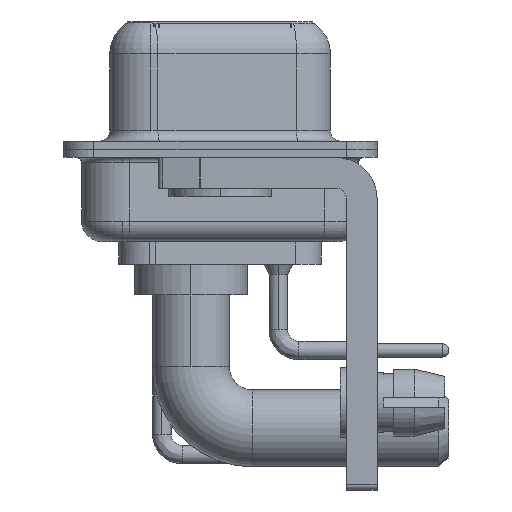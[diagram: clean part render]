
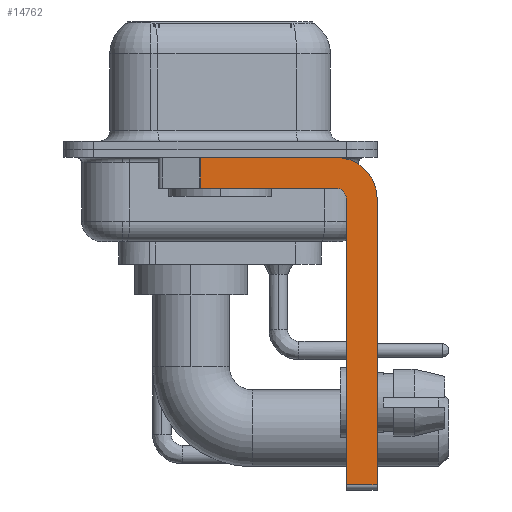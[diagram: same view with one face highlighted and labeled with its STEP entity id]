
A CAD part, left-side view. The second image highlights one B-rep face of the part: STEP entity #14762.
In plain terms, the highlighted planar face has unit normal (-1, 0, 0).
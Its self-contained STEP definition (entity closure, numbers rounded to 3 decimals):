
#224 = LINE ( 'NONE', #16806, #29640 ) ;
#698 = EDGE_CURVE ( 'NONE', #21235, #27137, #23874, .T. ) ;
#799 = ORIENTED_EDGE ( 'NONE', *, *, #13744, .F. ) ;
#1162 = EDGE_CURVE ( 'NONE', #33202, #16290, #27700, .T. ) ;
#1619 = AXIS2_PLACEMENT_3D ( 'NONE', #22233, #13235, #7358 ) ;
#1814 = ORIENTED_EDGE ( 'NONE', *, *, #33351, .T. ) ;
#1931 = CARTESIAN_POINT ( 'NONE',  ( -2.9, -5.65, -1.9 ) ) ;
#2592 = CARTESIAN_POINT ( 'NONE',  ( -2.9, -7.65, -2.4 ) ) ;
#2836 = CARTESIAN_POINT ( 'NONE',  ( -2.9, 0.978, -1.9 ) ) ;
#4672 = VECTOR ( 'NONE', #6950, 1000. ) ;
#6358 = VERTEX_POINT ( 'NONE', #12245 ) ;
#6875 = CARTESIAN_POINT ( 'NONE',  ( -2.9, -6.15, -16.35 ) ) ;
#6950 = DIRECTION ( 'NONE',  ( 0., 1., 0. ) ) ;
#7358 = DIRECTION ( 'NONE',  ( 0., 0., -1. ) ) ;
#7416 = DIRECTION ( 'NONE',  ( 0., -1., 0. ) ) ;
#8097 = VERTEX_POINT ( 'NONE', #25454 ) ;
#8476 = AXIS2_PLACEMENT_3D ( 'NONE', #9347, #26274, #34347 ) ;
#9347 = CARTESIAN_POINT ( 'NONE',  ( -2.9, -5.65, -2.4 ) ) ;
#10268 = EDGE_CURVE ( 'NONE', #16290, #21235, #20741, .T. ) ;
#10754 = VECTOR ( 'NONE', #27327, 1000. ) ;
#11011 = FACE_OUTER_BOUND ( 'NONE', #13887, .T. ) ;
#11871 = DIRECTION ( 'NONE',  ( 0., -1., 0. ) ) ;
#12245 = CARTESIAN_POINT ( 'NONE',  ( -2.9, 0.978, -0.4 ) ) ;
#12428 = EDGE_CURVE ( 'NONE', #6358, #27137, #224, .T. ) ;
#13235 = DIRECTION ( 'NONE',  ( 1., 0., 0. ) ) ;
#13590 = EDGE_CURVE ( 'NONE', #24526, #23836, #19670, .T. ) ;
#13744 = EDGE_CURVE ( 'NONE', #8097, #24526, #24337, .T. ) ;
#13887 = EDGE_LOOP ( 'NONE', ( #33103, #19713, #18801, #13941, #35571, #1814, #21103, #799 ) ) ;
#13941 = ORIENTED_EDGE ( 'NONE', *, *, #10268, .F. ) ;
#14249 = AXIS2_PLACEMENT_3D ( 'NONE', #33777, #14308, #25518 ) ;
#14308 = DIRECTION ( 'NONE',  ( -1., 0., 0. ) ) ;
#14762 = ADVANCED_FACE ( 'NONE', ( #11011 ), #27752, .F. ) ;
#16290 = VERTEX_POINT ( 'NONE', #27798 ) ;
#16806 = CARTESIAN_POINT ( 'NONE',  ( -2.9, 0.978, -1.9 ) ) ;
#17212 = LINE ( 'NONE', #22878, #17606 ) ;
#17606 = VECTOR ( 'NONE', #11871, 1000. ) ;
#18801 = ORIENTED_EDGE ( 'NONE', *, *, #698, .F. ) ;
#19670 = LINE ( 'NONE', #31049, #31983 ) ;
#19713 = ORIENTED_EDGE ( 'NONE', *, *, #12428, .T. ) ;
#20741 = CIRCLE ( 'NONE', #14249, 0.5 ) ;
#21103 = ORIENTED_EDGE ( 'NONE', *, *, #13590, .F. ) ;
#21235 = VERTEX_POINT ( 'NONE', #1931 ) ;
#21413 = LINE ( 'NONE', #32612, #25552 ) ;
#22233 = CARTESIAN_POINT ( 'NONE',  ( -2.9, -5.65, -2.4 ) ) ;
#22878 = CARTESIAN_POINT ( 'NONE',  ( -2.9, 3., -0.4 ) ) ;
#23836 = VERTEX_POINT ( 'NONE', #28754 ) ;
#23874 = LINE ( 'NONE', #29037, #4672 ) ;
#24337 = CIRCLE ( 'NONE', #8476, 2. ) ;
#24526 = VERTEX_POINT ( 'NONE', #2592 ) ;
#24767 = CARTESIAN_POINT ( 'NONE',  ( -2.9, -6.15, -16.6 ) ) ;
#25454 = CARTESIAN_POINT ( 'NONE',  ( -2.9, -5.65, -0.4 ) ) ;
#25518 = DIRECTION ( 'NONE',  ( 0., 0., 1. ) ) ;
#25552 = VECTOR ( 'NONE', #7416, 1000. ) ;
#25898 = EDGE_CURVE ( 'NONE', #6358, #8097, #17212, .T. ) ;
#26274 = DIRECTION ( 'NONE',  ( 1., 0., 0. ) ) ;
#27137 = VERTEX_POINT ( 'NONE', #2836 ) ;
#27327 = DIRECTION ( 'NONE',  ( 0., 0., 1. ) ) ;
#27700 = LINE ( 'NONE', #24767, #10754 ) ;
#27752 = PLANE ( 'NONE',  #1619 ) ;
#27798 = CARTESIAN_POINT ( 'NONE',  ( -2.9, -6.15, -2.4 ) ) ;
#28754 = CARTESIAN_POINT ( 'NONE',  ( -2.9, -7.65, -16.35 ) ) ;
#29037 = CARTESIAN_POINT ( 'NONE',  ( -2.9, -5.65, -1.9 ) ) ;
#29640 = VECTOR ( 'NONE', #30945, 1000. ) ;
#30945 = DIRECTION ( 'NONE',  ( 0., 0., -1. ) ) ;
#31049 = CARTESIAN_POINT ( 'NONE',  ( -2.9, -7.65, -2.4 ) ) ;
#31983 = VECTOR ( 'NONE', #33425, 1000. ) ;
#32612 = CARTESIAN_POINT ( 'NONE',  ( -2.9, -5.65, -16.35 ) ) ;
#33103 = ORIENTED_EDGE ( 'NONE', *, *, #25898, .F. ) ;
#33202 = VERTEX_POINT ( 'NONE', #6875 ) ;
#33351 = EDGE_CURVE ( 'NONE', #33202, #23836, #21413, .T. ) ;
#33425 = DIRECTION ( 'NONE',  ( 0., 0., -1. ) ) ;
#33777 = CARTESIAN_POINT ( 'NONE',  ( -2.9, -5.65, -2.4 ) ) ;
#34347 = DIRECTION ( 'NONE',  ( 0., 0., -1. ) ) ;
#35571 = ORIENTED_EDGE ( 'NONE', *, *, #1162, .F. ) ;
